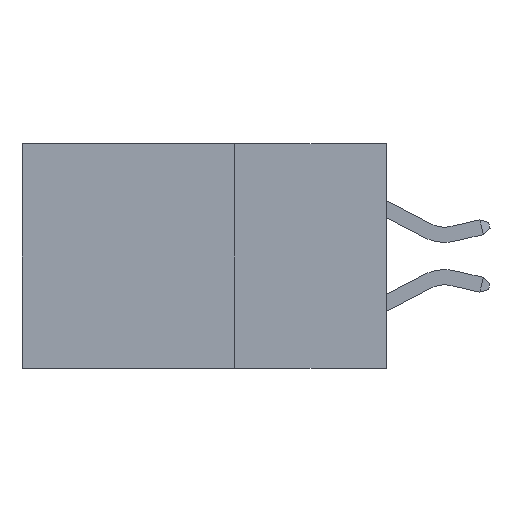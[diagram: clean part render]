
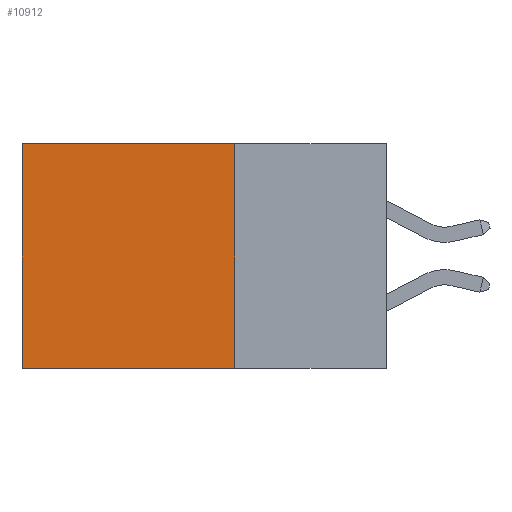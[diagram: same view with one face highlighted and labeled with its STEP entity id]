
A CAD part, left-side view. The second image highlights one B-rep face of the part: STEP entity #10912.
In plain terms, the highlighted planar face has unit normal (-1, 0, 0).
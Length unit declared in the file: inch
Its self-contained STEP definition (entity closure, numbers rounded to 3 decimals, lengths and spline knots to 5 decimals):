
#230 = VECTOR ( 'NONE', #17109, 39.37008 ) ;
#545 = CARTESIAN_POINT ( 'NONE',  ( 0.2615, 0.25, -0.37 ) ) ;
#1514 = EDGE_LOOP ( 'NONE', ( #18440, #17464, #9765, #15079 ) ) ;
#2022 = VERTEX_POINT ( 'NONE', #13463 ) ;
#2268 = DIRECTION ( 'NONE',  ( 1., 0., 0. ) ) ;
#2946 = LINE ( 'NONE', #4897, #13304 ) ;
#2997 = CARTESIAN_POINT ( 'NONE',  ( 0.2615, 0.6, -0.37 ) ) ;
#4333 = AXIS2_PLACEMENT_3D ( 'NONE', #8504, #2268, #16694 ) ;
#4897 = CARTESIAN_POINT ( 'NONE',  ( 0.2615, 0.25, 0. ) ) ;
#5139 = DIRECTION ( 'NONE',  ( 0., 0., -1. ) ) ;
#5275 = LINE ( 'NONE', #545, #230 ) ;
#5755 = VECTOR ( 'NONE', #5139, 39.37008 ) ;
#8191 = CARTESIAN_POINT ( 'NONE',  ( 0.2615, 0.6, 0. ) ) ;
#8504 = CARTESIAN_POINT ( 'NONE',  ( 0.2615, 0.25, -0.37 ) ) ;
#9692 = VECTOR ( 'NONE', #10229, 39.37008 ) ;
#9765 = ORIENTED_EDGE ( 'NONE', *, *, #25526, .F. ) ;
#10229 = DIRECTION ( 'NONE',  ( 0., 1., 0. ) ) ;
#10912 = ADVANCED_FACE ( 'NONE', ( #25822 ), #14654, .F. ) ;
#11077 = VERTEX_POINT ( 'NONE', #19201 ) ;
#13304 = VECTOR ( 'NONE', #25448, 39.37008 ) ;
#13463 = CARTESIAN_POINT ( 'NONE',  ( 0.2615, 0.25, -0.37 ) ) ;
#14654 = PLANE ( 'NONE',  #4333 ) ;
#15079 = ORIENTED_EDGE ( 'NONE', *, *, #15421, .T. ) ;
#15421 = EDGE_CURVE ( 'NONE', #17799, #20063, #2946, .T. ) ;
#16694 = DIRECTION ( 'NONE',  ( 0., 0., -1. ) ) ;
#17109 = DIRECTION ( 'NONE',  ( 0., 0., -1. ) ) ;
#17122 = EDGE_CURVE ( 'NONE', #2022, #11077, #21197, .T. ) ;
#17464 = ORIENTED_EDGE ( 'NONE', *, *, #17122, .F. ) ;
#17799 = VERTEX_POINT ( 'NONE', #22353 ) ;
#18180 = EDGE_CURVE ( 'NONE', #20063, #11077, #22103, .T. ) ;
#18440 = ORIENTED_EDGE ( 'NONE', *, *, #18180, .T. ) ;
#19201 = CARTESIAN_POINT ( 'NONE',  ( 0.2615, 0.6, -0.37 ) ) ;
#20063 = VERTEX_POINT ( 'NONE', #8191 ) ;
#20397 = CARTESIAN_POINT ( 'NONE',  ( 0.2615, 0.25, -0.37 ) ) ;
#21197 = LINE ( 'NONE', #20397, #9692 ) ;
#22103 = LINE ( 'NONE', #2997, #5755 ) ;
#22353 = CARTESIAN_POINT ( 'NONE',  ( 0.2615, 0.25, 0. ) ) ;
#25448 = DIRECTION ( 'NONE',  ( 0., 1., 0. ) ) ;
#25526 = EDGE_CURVE ( 'NONE', #17799, #2022, #5275, .T. ) ;
#25822 = FACE_OUTER_BOUND ( 'NONE', #1514, .T. ) ;
